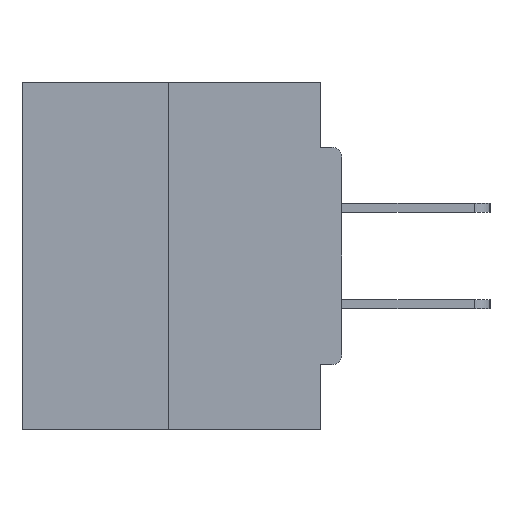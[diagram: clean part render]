
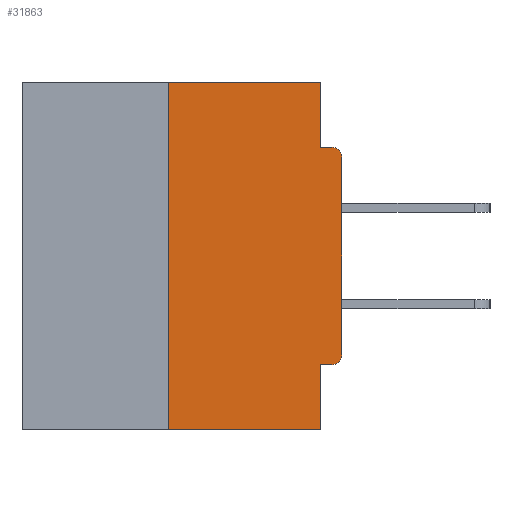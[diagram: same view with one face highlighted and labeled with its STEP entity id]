
A CAD part, left-side view. The second image highlights one B-rep face of the part: STEP entity #31863.
In plain terms, the highlighted planar face has unit normal (-1, 0, 0).
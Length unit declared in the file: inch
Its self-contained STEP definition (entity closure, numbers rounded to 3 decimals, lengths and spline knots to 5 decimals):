
#1342 = VERTEX_POINT ( 'NONE', #10790 ) ;
#1489 = EDGE_CURVE ( 'NONE', #1948, #29994, #17802, .T. ) ;
#1543 = LINE ( 'NONE', #11864, #6978 ) ;
#1948 = VERTEX_POINT ( 'NONE', #28866 ) ;
#2175 = VECTOR ( 'NONE', #30856, 39.37008 ) ;
#2875 = DIRECTION ( 'NONE',  ( 0., 0., 1. ) ) ;
#3349 = CARTESIAN_POINT ( 'NONE',  ( 0., 0., -0.4065 ) ) ;
#3518 = CARTESIAN_POINT ( 'NONE',  ( 0., 0.46, 0. ) ) ;
#3820 = DIRECTION ( 'NONE',  ( 0., 0., -1. ) ) ;
#4181 = VERTEX_POINT ( 'NONE', #16293 ) ;
#5444 = ORIENTED_EDGE ( 'NONE', *, *, #28424, .T. ) ;
#5740 = VECTOR ( 'NONE', #8142, 39.37008 ) ;
#6817 = VERTEX_POINT ( 'NONE', #18902 ) ;
#6978 = VECTOR ( 'NONE', #31843, 39.37008 ) ;
#7002 = ORIENTED_EDGE ( 'NONE', *, *, #28248, .T. ) ;
#7546 = VERTEX_POINT ( 'NONE', #27118 ) ;
#8142 = DIRECTION ( 'NONE',  ( 0., 0., 1. ) ) ;
#8539 = VECTOR ( 'NONE', #13529, 39.37008 ) ;
#9227 = VERTEX_POINT ( 'NONE', #21284 ) ;
#9333 = DIRECTION ( 'NONE',  ( -1., 0., 0. ) ) ;
#9676 = EDGE_CURVE ( 'NONE', #1342, #29297, #30013, .T. ) ;
#10485 = PLANE ( 'NONE',  #18835 ) ;
#10790 = CARTESIAN_POINT ( 'NONE',  ( 0., 0.25, -0.5 ) ) ;
#10842 = CARTESIAN_POINT ( 'NONE',  ( 0., 0.031, -0.0935 ) ) ;
#11115 = VECTOR ( 'NONE', #2875, 39.37008 ) ;
#11626 = AXIS2_PLACEMENT_3D ( 'NONE', #13107, #25777, #23503 ) ;
#11807 = EDGE_CURVE ( 'NONE', #4181, #21520, #20186, .T. ) ;
#11864 = CARTESIAN_POINT ( 'NONE',  ( 0., 0.031, -0.5 ) ) ;
#12487 = ORIENTED_EDGE ( 'NONE', *, *, #17462, .F. ) ;
#12694 = CARTESIAN_POINT ( 'NONE',  ( 0., 0., 0. ) ) ;
#12991 = DIRECTION ( 'NONE',  ( 0., 1., 0. ) ) ;
#13107 = CARTESIAN_POINT ( 'NONE',  ( 0., 0.015, -0.3915 ) ) ;
#13529 = DIRECTION ( 'NONE',  ( 0., -1., 0. ) ) ;
#13755 = LINE ( 'NONE', #3349, #27831 ) ;
#14375 = EDGE_CURVE ( 'NONE', #29994, #21520, #26652, .T. ) ;
#14661 = LINE ( 'NONE', #12694, #11115 ) ;
#14970 = CARTESIAN_POINT ( 'NONE',  ( 0., 0.031, -0.5 ) ) ;
#15648 = EDGE_CURVE ( 'NONE', #9227, #24131, #1543, .T. ) ;
#16219 = CARTESIAN_POINT ( 'NONE',  ( 0., 0.25, 0. ) ) ;
#16293 = CARTESIAN_POINT ( 'NONE',  ( 0., 0., -0.1085 ) ) ;
#16790 = ORIENTED_EDGE ( 'NONE', *, *, #27531, .F. ) ;
#17462 = EDGE_CURVE ( 'NONE', #29297, #1948, #18691, .T. ) ;
#17763 = ORIENTED_EDGE ( 'NONE', *, *, #15648, .F. ) ;
#17802 = LINE ( 'NONE', #31774, #2175 ) ;
#18691 = LINE ( 'NONE', #22751, #25335 ) ;
#18835 = AXIS2_PLACEMENT_3D ( 'NONE', #3518, #31245, #3820 ) ;
#18902 = CARTESIAN_POINT ( 'NONE',  ( 0., 0., -0.3915 ) ) ;
#19111 = DIRECTION ( 'NONE',  ( 0., 0., -1. ) ) ;
#19541 = ORIENTED_EDGE ( 'NONE', *, *, #31652, .T. ) ;
#20037 = VECTOR ( 'NONE', #27070, 39.37008 ) ;
#20186 = CIRCLE ( 'NONE', #29864, 0.015 ) ;
#20868 = ORIENTED_EDGE ( 'NONE', *, *, #9676, .F. ) ;
#21102 = LINE ( 'NONE', #23925, #8539 ) ;
#21284 = CARTESIAN_POINT ( 'NONE',  ( 0., 0.031, -0.4065 ) ) ;
#21383 = EDGE_LOOP ( 'NONE', ( #12487, #20868, #5444, #17763, #16790, #7002, #19541, #30458, #28455, #31036 ) ) ;
#21520 = VERTEX_POINT ( 'NONE', #27183 ) ;
#21687 = FACE_OUTER_BOUND ( 'NONE', #21383, .T. ) ;
#21728 = CARTESIAN_POINT ( 'NONE',  ( 0., 0., -0.0935 ) ) ;
#22751 = CARTESIAN_POINT ( 'NONE',  ( 0., 0.46, 0. ) ) ;
#23091 = CIRCLE ( 'NONE', #11626, 0.015 ) ;
#23503 = DIRECTION ( 'NONE',  ( 0., 0., -1. ) ) ;
#23925 = CARTESIAN_POINT ( 'NONE',  ( 0., 0.46, -0.5 ) ) ;
#24131 = VERTEX_POINT ( 'NONE', #14970 ) ;
#25171 = DIRECTION ( 'NONE',  ( 0., -1., 0. ) ) ;
#25335 = VECTOR ( 'NONE', #25171, 39.37008 ) ;
#25654 = CARTESIAN_POINT ( 'NONE',  ( 0., 0.25, 0. ) ) ;
#25777 = DIRECTION ( 'NONE',  ( -1., 0., 0. ) ) ;
#26652 = LINE ( 'NONE', #21728, #20037 ) ;
#27070 = DIRECTION ( 'NONE',  ( 0., -1., 0. ) ) ;
#27118 = CARTESIAN_POINT ( 'NONE',  ( 0., 0.015, -0.4065 ) ) ;
#27183 = CARTESIAN_POINT ( 'NONE',  ( 0., 0.015, -0.0935 ) ) ;
#27531 = EDGE_CURVE ( 'NONE', #7546, #9227, #13755, .T. ) ;
#27831 = VECTOR ( 'NONE', #12991, 39.37008 ) ;
#28248 = EDGE_CURVE ( 'NONE', #7546, #6817, #23091, .T. ) ;
#28424 = EDGE_CURVE ( 'NONE', #1342, #24131, #21102, .T. ) ;
#28455 = ORIENTED_EDGE ( 'NONE', *, *, #14375, .F. ) ;
#28866 = CARTESIAN_POINT ( 'NONE',  ( 0., 0.031, 0. ) ) ;
#29116 = CARTESIAN_POINT ( 'NONE',  ( 0., 0.015, -0.1085 ) ) ;
#29297 = VERTEX_POINT ( 'NONE', #16219 ) ;
#29864 = AXIS2_PLACEMENT_3D ( 'NONE', #29116, #9333, #19111 ) ;
#29994 = VERTEX_POINT ( 'NONE', #10842 ) ;
#30013 = LINE ( 'NONE', #25654, #5740 ) ;
#30458 = ORIENTED_EDGE ( 'NONE', *, *, #11807, .T. ) ;
#30856 = DIRECTION ( 'NONE',  ( 0., 0., -1. ) ) ;
#31036 = ORIENTED_EDGE ( 'NONE', *, *, #1489, .F. ) ;
#31245 = DIRECTION ( 'NONE',  ( 1., 0., 0. ) ) ;
#31652 = EDGE_CURVE ( 'NONE', #6817, #4181, #14661, .T. ) ;
#31774 = CARTESIAN_POINT ( 'NONE',  ( 0., 0.031, 0. ) ) ;
#31843 = DIRECTION ( 'NONE',  ( 0., 0., -1. ) ) ;
#31863 = ADVANCED_FACE ( 'NONE', ( #21687 ), #10485, .F. ) ;
